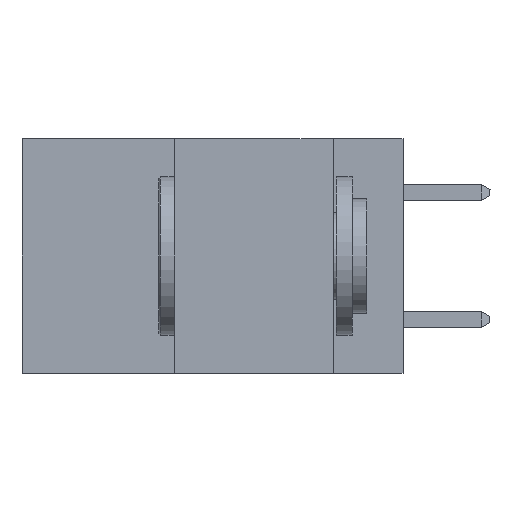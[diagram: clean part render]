
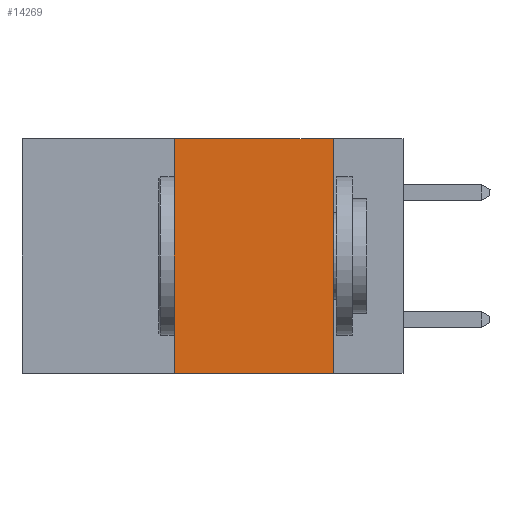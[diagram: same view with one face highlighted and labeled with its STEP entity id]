
A CAD part, left-side view. The second image highlights one B-rep face of the part: STEP entity #14269.
In plain terms, the highlighted planar face has unit normal (-1, 0, 0).
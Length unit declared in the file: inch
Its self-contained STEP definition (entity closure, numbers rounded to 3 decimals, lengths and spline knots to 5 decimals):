
#377 = ORIENTED_EDGE ( 'NONE', *, *, #3811, .F. ) ;
#410 = LINE ( 'NONE', #13300, #6464 ) ;
#451 = DIRECTION ( 'NONE',  ( 0., 0., 1. ) ) ;
#1285 = CARTESIAN_POINT ( 'NONE',  ( 0., 0.6, 0. ) ) ;
#1306 = CARTESIAN_POINT ( 'NONE',  ( 0., 0.6, 0. ) ) ;
#1445 = DIRECTION ( 'NONE',  ( 0., 0., -1. ) ) ;
#1778 = EDGE_CURVE ( 'NONE', #4078, #3792, #12875, .T. ) ;
#2446 = DIRECTION ( 'NONE',  ( 0., -1., 0. ) ) ;
#2662 = ORIENTED_EDGE ( 'NONE', *, *, #7611, .T. ) ;
#2671 = DIRECTION ( 'NONE',  ( 0., -1., 0. ) ) ;
#3063 = VECTOR ( 'NONE', #1445, 39.37008 ) ;
#3770 = CARTESIAN_POINT ( 'NONE',  ( 0., 0.11, 0. ) ) ;
#3792 = VERTEX_POINT ( 'NONE', #14834 ) ;
#3811 = EDGE_CURVE ( 'NONE', #6140, #4078, #15202, .T. ) ;
#4078 = VERTEX_POINT ( 'NONE', #8262 ) ;
#4255 = VECTOR ( 'NONE', #2446, 39.37008 ) ;
#6140 = VERTEX_POINT ( 'NONE', #8836 ) ;
#6464 = VECTOR ( 'NONE', #2671, 39.37008 ) ;
#6606 = EDGE_CURVE ( 'NONE', #3792, #11393, #14342, .T. ) ;
#6772 = ORIENTED_EDGE ( 'NONE', *, *, #6606, .F. ) ;
#7310 = FACE_OUTER_BOUND ( 'NONE', #13351, .T. ) ;
#7611 = EDGE_CURVE ( 'NONE', #6140, #11393, #410, .T. ) ;
#7691 = CARTESIAN_POINT ( 'NONE',  ( 0., 0.36, 0. ) ) ;
#8262 = CARTESIAN_POINT ( 'NONE',  ( 0., 0.36, 0. ) ) ;
#8440 = DIRECTION ( 'NONE',  ( 0., 0., -1. ) ) ;
#8778 = ORIENTED_EDGE ( 'NONE', *, *, #1778, .F. ) ;
#8836 = CARTESIAN_POINT ( 'NONE',  ( 0., 0.36, -0.37 ) ) ;
#9602 = CARTESIAN_POINT ( 'NONE',  ( 0., 0.11, -0.37 ) ) ;
#10779 = PLANE ( 'NONE',  #13975 ) ;
#11393 = VERTEX_POINT ( 'NONE', #9602 ) ;
#12006 = VECTOR ( 'NONE', #451, 39.37008 ) ;
#12875 = LINE ( 'NONE', #1285, #4255 ) ;
#13147 = DIRECTION ( 'NONE',  ( 1., 0., 0. ) ) ;
#13300 = CARTESIAN_POINT ( 'NONE',  ( 0., 0.6, -0.37 ) ) ;
#13351 = EDGE_LOOP ( 'NONE', ( #6772, #8778, #377, #2662 ) ) ;
#13975 = AXIS2_PLACEMENT_3D ( 'NONE', #1306, #13147, #8440 ) ;
#14269 = ADVANCED_FACE ( 'NONE', ( #7310 ), #10779, .F. ) ;
#14342 = LINE ( 'NONE', #3770, #3063 ) ;
#14834 = CARTESIAN_POINT ( 'NONE',  ( 0., 0.11, 0. ) ) ;
#15202 = LINE ( 'NONE', #7691, #12006 ) ;
